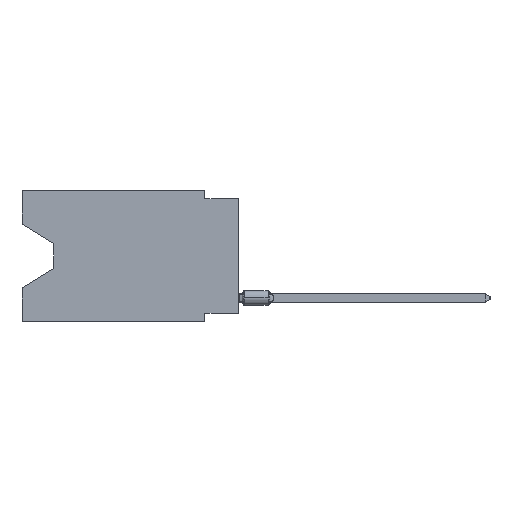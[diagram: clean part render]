
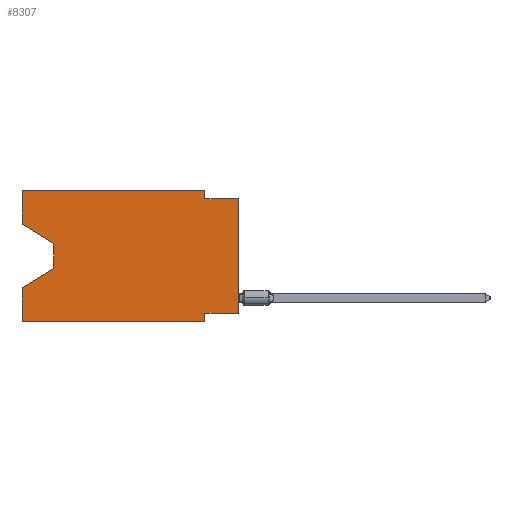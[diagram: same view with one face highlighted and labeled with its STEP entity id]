
A CAD part, left-side view. The second image highlights one B-rep face of the part: STEP entity #8307.
In plain terms, the highlighted planar face has unit normal (-1, 0, 0).
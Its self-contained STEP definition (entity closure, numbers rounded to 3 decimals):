
#88 = EDGE_CURVE ( 'NONE', #22313, #64774, #43689, .T. ) ;
#234 = VECTOR ( 'NONE', #9276, 1000. ) ;
#285 = CARTESIAN_POINT ( 'NONE',  ( 0., 16.383, -7.36 ) ) ;
#2770 = CARTESIAN_POINT ( 'NONE',  ( 0., 0., 0. ) ) ;
#3145 = LINE ( 'NONE', #2770, #234 ) ;
#4181 = CARTESIAN_POINT ( 'NONE',  ( 0., 2.54, 0. ) ) ;
#5426 = VECTOR ( 'NONE', #25264, 1000. ) ;
#6150 = ORIENTED_EDGE ( 'NONE', *, *, #7639, .T. ) ;
#6745 = VERTEX_POINT ( 'NONE', #73317 ) ;
#7174 = CARTESIAN_POINT ( 'NONE',  ( 0., 2.54, -9.906 ) ) ;
#7639 = EDGE_CURVE ( 'NONE', #30508, #36613, #58034, .T. ) ;
#8307 = ADVANCED_FACE ( 'NONE', ( #32202 ), #31071, .F. ) ;
#9272 = CARTESIAN_POINT ( 'NONE',  ( 0., 2.54, -9.271 ) ) ;
#9276 = DIRECTION ( 'NONE',  ( 0., 0., 1. ) ) ;
#10765 = EDGE_CURVE ( 'NONE', #12899, #13436, #65450, .T. ) ;
#11928 = VECTOR ( 'NONE', #59492, 1000. ) ;
#12899 = VERTEX_POINT ( 'NONE', #23864 ) ;
#13436 = VERTEX_POINT ( 'NONE', #4181 ) ;
#13584 = EDGE_CURVE ( 'NONE', #40939, #32582, #47044, .T. ) ;
#14949 = VECTOR ( 'NONE', #28178, 1000. ) ;
#15458 = VECTOR ( 'NONE', #62302, 1000. ) ;
#16687 = CARTESIAN_POINT ( 'NONE',  ( 0., 0., -0.635 ) ) ;
#16851 = ORIENTED_EDGE ( 'NONE', *, *, #58692, .T. ) ;
#17356 = CARTESIAN_POINT ( 'NONE',  ( 0., 16.383, 0. ) ) ;
#17851 = CARTESIAN_POINT ( 'NONE',  ( 0., 13.97, -5.893 ) ) ;
#18407 = CARTESIAN_POINT ( 'NONE',  ( 0., 2.54, -9.906 ) ) ;
#18498 = VECTOR ( 'NONE', #29551, 1000. ) ;
#18787 = CARTESIAN_POINT ( 'NONE',  ( 0., 16.383, -9.906 ) ) ;
#20249 = VECTOR ( 'NONE', #37913, 1000. ) ;
#20288 = LINE ( 'NONE', #49788, #20249 ) ;
#21239 = LINE ( 'NONE', #18407, #5426 ) ;
#21683 = ORIENTED_EDGE ( 'NONE', *, *, #48658, .F. ) ;
#21872 = ORIENTED_EDGE ( 'NONE', *, *, #13584, .F. ) ;
#21976 = CARTESIAN_POINT ( 'NONE',  ( 0., 0., -0.635 ) ) ;
#22313 = VERTEX_POINT ( 'NONE', #17851 ) ;
#22891 = ORIENTED_EDGE ( 'NONE', *, *, #53822, .F. ) ;
#23000 = LINE ( 'NONE', #35601, #25265 ) ;
#23170 = CARTESIAN_POINT ( 'NONE',  ( 0., 16.383, -9.906 ) ) ;
#23289 = EDGE_CURVE ( 'NONE', #13436, #67831, #20288, .T. ) ;
#23298 = DIRECTION ( 'NONE',  ( 0., 1., 0. ) ) ;
#23864 = CARTESIAN_POINT ( 'NONE',  ( 0., 16.383, 0. ) ) ;
#25264 = DIRECTION ( 'NONE',  ( 0., 0., -1. ) ) ;
#25265 = VECTOR ( 'NONE', #64004, 1000. ) ;
#25524 = AXIS2_PLACEMENT_3D ( 'NONE', #54431, #73240, #48688 ) ;
#25549 = VECTOR ( 'NONE', #31439, 1000. ) ;
#28178 = DIRECTION ( 'NONE',  ( 0., -1., 0. ) ) ;
#29551 = DIRECTION ( 'NONE',  ( 0., 0., -1. ) ) ;
#29703 = ORIENTED_EDGE ( 'NONE', *, *, #23289, .F. ) ;
#30508 = VERTEX_POINT ( 'NONE', #18787 ) ;
#31071 = PLANE ( 'NONE',  #25524 ) ;
#31439 = DIRECTION ( 'NONE',  ( 0., 0., 1. ) ) ;
#31565 = VERTEX_POINT ( 'NONE', #60233 ) ;
#32202 = FACE_OUTER_BOUND ( 'NONE', #35772, .T. ) ;
#32582 = VERTEX_POINT ( 'NONE', #9272 ) ;
#35601 = CARTESIAN_POINT ( 'NONE',  ( 0., 16.383, -2.546 ) ) ;
#35660 = CARTESIAN_POINT ( 'NONE',  ( 0., 13.97, -4.013 ) ) ;
#35772 = EDGE_LOOP ( 'NONE', ( #55088, #16851, #53097, #22891, #6150, #21683, #21872, #72503, #59143, #29703, #50105, #63602 ) ) ;
#36012 = EDGE_CURVE ( 'NONE', #6745, #31565, #23000, .T. ) ;
#36613 = VERTEX_POINT ( 'NONE', #7174 ) ;
#36688 = DIRECTION ( 'NONE',  ( 0., -1., 0. ) ) ;
#37156 = VERTEX_POINT ( 'NONE', #21976 ) ;
#37570 = CARTESIAN_POINT ( 'NONE',  ( 0., 13.97, -5.893 ) ) ;
#37913 = DIRECTION ( 'NONE',  ( 0., 0., -1. ) ) ;
#38924 = LINE ( 'NONE', #16687, #14949 ) ;
#40939 = VERTEX_POINT ( 'NONE', #41606 ) ;
#40951 = VECTOR ( 'NONE', #36688, 1000. ) ;
#41606 = CARTESIAN_POINT ( 'NONE',  ( 0., 0., -9.271 ) ) ;
#42189 = LINE ( 'NONE', #42933, #25549 ) ;
#42933 = CARTESIAN_POINT ( 'NONE',  ( 0., 16.383, 0. ) ) ;
#43689 = LINE ( 'NONE', #37570, #74616 ) ;
#46927 = DIRECTION ( 'NONE',  ( 0., 0.855, -0.519 ) ) ;
#47044 = LINE ( 'NONE', #64685, #52113 ) ;
#48658 = EDGE_CURVE ( 'NONE', #32582, #36613, #21239, .T. ) ;
#48688 = DIRECTION ( 'NONE',  ( 0., 0., -1. ) ) ;
#49788 = CARTESIAN_POINT ( 'NONE',  ( 0., 2.54, 0. ) ) ;
#50105 = ORIENTED_EDGE ( 'NONE', *, *, #10765, .F. ) ;
#52113 = VECTOR ( 'NONE', #23298, 1000. ) ;
#53097 = ORIENTED_EDGE ( 'NONE', *, *, #88, .T. ) ;
#53822 = EDGE_CURVE ( 'NONE', #30508, #64774, #42189, .T. ) ;
#54431 = CARTESIAN_POINT ( 'NONE',  ( 0., 16.383, 0. ) ) ;
#55088 = ORIENTED_EDGE ( 'NONE', *, *, #36012, .T. ) ;
#57928 = LINE ( 'NONE', #35660, #18498 ) ;
#58034 = LINE ( 'NONE', #23170, #15458 ) ;
#58692 = EDGE_CURVE ( 'NONE', #31565, #22313, #57928, .T. ) ;
#59143 = ORIENTED_EDGE ( 'NONE', *, *, #64987, .F. ) ;
#59250 = EDGE_CURVE ( 'NONE', #40939, #37156, #3145, .T. ) ;
#59492 = DIRECTION ( 'NONE',  ( 0., 0., 1. ) ) ;
#60233 = CARTESIAN_POINT ( 'NONE',  ( 0., 13.97, -4.013 ) ) ;
#60746 = CARTESIAN_POINT ( 'NONE',  ( 0., 2.54, -0.635 ) ) ;
#62302 = DIRECTION ( 'NONE',  ( 0., -1., 0. ) ) ;
#63602 = ORIENTED_EDGE ( 'NONE', *, *, #73145, .F. ) ;
#64004 = DIRECTION ( 'NONE',  ( 0., -0.855, -0.519 ) ) ;
#64685 = CARTESIAN_POINT ( 'NONE',  ( 0., 0., -9.271 ) ) ;
#64774 = VERTEX_POINT ( 'NONE', #285 ) ;
#64987 = EDGE_CURVE ( 'NONE', #67831, #37156, #38924, .T. ) ;
#65450 = LINE ( 'NONE', #71224, #40951 ) ;
#67831 = VERTEX_POINT ( 'NONE', #60746 ) ;
#69881 = LINE ( 'NONE', #17356, #11928 ) ;
#71224 = CARTESIAN_POINT ( 'NONE',  ( 0., 16.383, 0. ) ) ;
#72503 = ORIENTED_EDGE ( 'NONE', *, *, #59250, .T. ) ;
#73145 = EDGE_CURVE ( 'NONE', #6745, #12899, #69881, .T. ) ;
#73240 = DIRECTION ( 'NONE',  ( 1., 0., 0. ) ) ;
#73317 = CARTESIAN_POINT ( 'NONE',  ( 0., 16.383, -2.546 ) ) ;
#74616 = VECTOR ( 'NONE', #46927, 1000. ) ;
